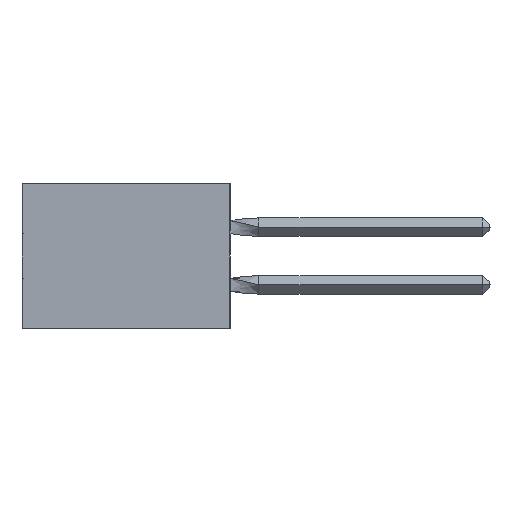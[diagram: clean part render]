
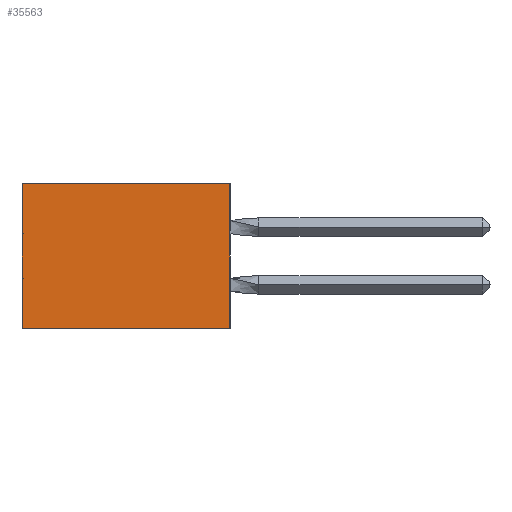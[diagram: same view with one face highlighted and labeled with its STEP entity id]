
A CAD part, left-side view. The second image highlights one B-rep face of the part: STEP entity #35563.
In plain terms, the highlighted planar face has unit normal (-1, 0, 0).
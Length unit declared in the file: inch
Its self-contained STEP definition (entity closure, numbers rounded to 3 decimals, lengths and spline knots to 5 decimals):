
#2443 = DIRECTION ( 'NONE',  ( 0., 1., 0. ) ) ;
#3433 = EDGE_CURVE ( 'NONE', #11208, #10513, #40447, .T. ) ;
#4170 = EDGE_CURVE ( 'NONE', #10513, #43513, #14550, .T. ) ;
#5271 = DIRECTION ( 'NONE',  ( 0., 1., 0. ) ) ;
#5426 = CARTESIAN_POINT ( 'NONE',  ( 0.305, 0., -0.5 ) ) ;
#6084 = DIRECTION ( 'NONE',  ( 0., 0., -1. ) ) ;
#7397 = CARTESIAN_POINT ( 'NONE',  ( 0.305, 0.72, 0. ) ) ;
#7604 = DIRECTION ( 'NONE',  ( 0., 0., -1. ) ) ;
#7932 = CARTESIAN_POINT ( 'NONE',  ( 0.305, 0.72, -0.5 ) ) ;
#8809 = ORIENTED_EDGE ( 'NONE', *, *, #44695, .F. ) ;
#10513 = VERTEX_POINT ( 'NONE', #7397 ) ;
#10789 = CARTESIAN_POINT ( 'NONE',  ( 0.305, 0.72, -0.5 ) ) ;
#11208 = VERTEX_POINT ( 'NONE', #44504 ) ;
#14550 = LINE ( 'NONE', #7932, #16967 ) ;
#16750 = VERTEX_POINT ( 'NONE', #35691 ) ;
#16967 = VECTOR ( 'NONE', #7604, 39.37008 ) ;
#17105 = DIRECTION ( 'NONE',  ( 0., 0., -1. ) ) ;
#19157 = VECTOR ( 'NONE', #5271, 39.37008 ) ;
#19974 = PLANE ( 'NONE',  #37343 ) ;
#21714 = LINE ( 'NONE', #44307, #39118 ) ;
#23880 = CARTESIAN_POINT ( 'NONE',  ( 0.305, 0., -0.5 ) ) ;
#26900 = EDGE_CURVE ( 'NONE', #11208, #16750, #21714, .T. ) ;
#29691 = ORIENTED_EDGE ( 'NONE', *, *, #3433, .T. ) ;
#31484 = VECTOR ( 'NONE', #2443, 39.37008 ) ;
#33860 = ORIENTED_EDGE ( 'NONE', *, *, #26900, .F. ) ;
#35563 = ADVANCED_FACE ( 'NONE', ( #49081 ), #19974, .F. ) ;
#35691 = CARTESIAN_POINT ( 'NONE',  ( 0.305, 0., -0.5 ) ) ;
#37343 = AXIS2_PLACEMENT_3D ( 'NONE', #23880, #40920, #6084 ) ;
#39118 = VECTOR ( 'NONE', #17105, 39.37008 ) ;
#40109 = ORIENTED_EDGE ( 'NONE', *, *, #4170, .T. ) ;
#40447 = LINE ( 'NONE', #44359, #31484 ) ;
#40920 = DIRECTION ( 'NONE',  ( 1., 0., 0. ) ) ;
#43513 = VERTEX_POINT ( 'NONE', #10789 ) ;
#44307 = CARTESIAN_POINT ( 'NONE',  ( 0.305, 0., -0.5 ) ) ;
#44359 = CARTESIAN_POINT ( 'NONE',  ( 0.305, 0., 0. ) ) ;
#44504 = CARTESIAN_POINT ( 'NONE',  ( 0.305, 0., 0. ) ) ;
#44695 = EDGE_CURVE ( 'NONE', #16750, #43513, #46844, .T. ) ;
#46844 = LINE ( 'NONE', #5426, #19157 ) ;
#49081 = FACE_OUTER_BOUND ( 'NONE', #49086, .T. ) ;
#49086 = EDGE_LOOP ( 'NONE', ( #40109, #8809, #33860, #29691 ) ) ;
